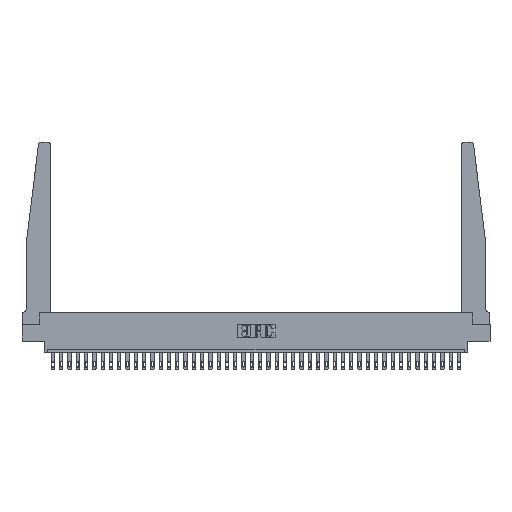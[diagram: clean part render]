
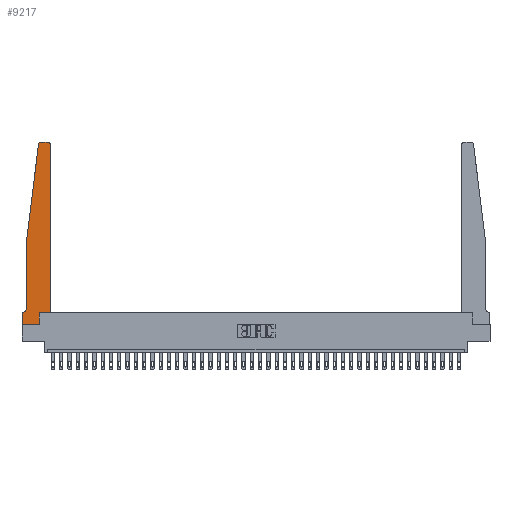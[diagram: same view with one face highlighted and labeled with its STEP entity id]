
A CAD part, top view. The second image highlights one B-rep face of the part: STEP entity #9217.
In plain terms, the highlighted planar face has unit normal (0, 0, 1).
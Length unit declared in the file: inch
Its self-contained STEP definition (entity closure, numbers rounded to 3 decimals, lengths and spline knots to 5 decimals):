
#181 = CARTESIAN_POINT ( 'NONE',  ( 0., 0.1875, 0.37 ) ) ;
#555 = LINE ( 'NONE', #16792, #15734 ) ;
#572 = VECTOR ( 'NONE', #16360, 39.37008 ) ;
#997 = CARTESIAN_POINT ( 'NONE',  ( 0.065, 1.25, 0.37 ) ) ;
#1011 = CARTESIAN_POINT ( 'NONE',  ( 0.065, 1.25, 0.37 ) ) ;
#1028 = EDGE_CURVE ( 'NONE', #31567, #10214, #10634, .T. ) ;
#1220 = CIRCLE ( 'NONE', #5780, 0.05 ) ;
#2375 = DIRECTION ( 'NONE',  ( 0., 0., 1. ) ) ;
#2556 = FACE_OUTER_BOUND ( 'NONE', #14897, .T. ) ;
#3318 = AXIS2_PLACEMENT_3D ( 'NONE', #9320, #3433, #23053 ) ;
#3376 = VERTEX_POINT ( 'NONE', #28971 ) ;
#3433 = DIRECTION ( 'NONE',  ( 0., 0., 1. ) ) ;
#4507 = LINE ( 'NONE', #18245, #8999 ) ;
#4530 = VECTOR ( 'NONE', #7963, 39.37008 ) ;
#4938 = EDGE_CURVE ( 'NONE', #9358, #31567, #4507, .T. ) ;
#5221 = CARTESIAN_POINT ( 'NONE',  ( 0.425, 2.72, 0.37 ) ) ;
#5393 = CARTESIAN_POINT ( 'NONE',  ( 0., 0.1875, 0.37 ) ) ;
#5651 = LINE ( 'NONE', #24561, #572 ) ;
#5780 = AXIS2_PLACEMENT_3D ( 'NONE', #29768, #18729, #18553 ) ;
#5893 = VERTEX_POINT ( 'NONE', #20055 ) ;
#6182 = ORIENTED_EDGE ( 'NONE', *, *, #1028, .T. ) ;
#6592 = EDGE_CURVE ( 'NONE', #24943, #9358, #1220, .T. ) ;
#7031 = VECTOR ( 'NONE', #18552, 39.37008 ) ;
#7167 = EDGE_CURVE ( 'NONE', #33819, #31018, #16520, .T. ) ;
#7266 = VERTEX_POINT ( 'NONE', #33075 ) ;
#7407 = VERTEX_POINT ( 'NONE', #25980 ) ;
#7668 = CARTESIAN_POINT ( 'NONE',  ( 0., 0., 0.37 ) ) ;
#7848 = LINE ( 'NONE', #7668, #7031 ) ;
#7963 = DIRECTION ( 'NONE',  ( -1., 0., 0. ) ) ;
#8357 = ORIENTED_EDGE ( 'NONE', *, *, #7167, .T. ) ;
#8999 = VECTOR ( 'NONE', #17708, 39.37008 ) ;
#9217 = ADVANCED_FACE ( 'NONE', ( #2556 ), #34974, .T. ) ;
#9297 = CARTESIAN_POINT ( 'NONE',  ( 0.065, 0.2375, 0.37 ) ) ;
#9320 = CARTESIAN_POINT ( 'NONE',  ( 0.27653, 2.72, 0.37 ) ) ;
#9358 = VERTEX_POINT ( 'NONE', #19488 ) ;
#9427 = DIRECTION ( 'NONE',  ( 0., -1., 0. ) ) ;
#9980 = ORIENTED_EDGE ( 'NONE', *, *, #11838, .T. ) ;
#10214 = VERTEX_POINT ( 'NONE', #28322 ) ;
#10397 = EDGE_CURVE ( 'NONE', #7266, #29901, #32520, .T. ) ;
#10634 = LINE ( 'NONE', #22047, #28386 ) ;
#11352 = DIRECTION ( 'NONE',  ( -0.122, -0.992, 0. ) ) ;
#11838 = EDGE_CURVE ( 'NONE', #5893, #7266, #5651, .T. ) ;
#12269 = LINE ( 'NONE', #28496, #30756 ) ;
#13611 = VECTOR ( 'NONE', #19169, 39.37008 ) ;
#14116 = AXIS2_PLACEMENT_3D ( 'NONE', #5393, #2375, #21468 ) ;
#14897 = EDGE_LOOP ( 'NONE', ( #18234, #28233, #8357, #33748, #35185, #18676, #6182, #30345, #31590, #9980, #26647, #16598 ) ) ;
#15734 = VECTOR ( 'NONE', #21629, 39.37008 ) ;
#16316 = CARTESIAN_POINT ( 'NONE',  ( 0.425, 0.18, 0.37 ) ) ;
#16360 = DIRECTION ( 'NONE',  ( 1., 0., 0. ) ) ;
#16520 = LINE ( 'NONE', #997, #17041 ) ;
#16598 = ORIENTED_EDGE ( 'NONE', *, *, #24276, .T. ) ;
#16792 = CARTESIAN_POINT ( 'NONE',  ( 0.2605, 0.18, 0.37 ) ) ;
#17041 = VECTOR ( 'NONE', #11352, 39.37008 ) ;
#17708 = DIRECTION ( 'NONE',  ( -1., 0., 0. ) ) ;
#18234 = ORIENTED_EDGE ( 'NONE', *, *, #32418, .T. ) ;
#18245 = CARTESIAN_POINT ( 'NONE',  ( 0.065, 0.1875, 0.37 ) ) ;
#18552 = DIRECTION ( 'NONE',  ( 1., 0., 0. ) ) ;
#18553 = DIRECTION ( 'NONE',  ( -1., 0., 0. ) ) ;
#18676 = ORIENTED_EDGE ( 'NONE', *, *, #4938, .T. ) ;
#18729 = DIRECTION ( 'NONE',  ( 0., 0., -1. ) ) ;
#19022 = AXIS2_PLACEMENT_3D ( 'NONE', #23329, #34876, #26531 ) ;
#19169 = DIRECTION ( 'NONE',  ( 0., 1., 0. ) ) ;
#19190 = DIRECTION ( 'NONE',  ( 0., -1., 0. ) ) ;
#19488 = CARTESIAN_POINT ( 'NONE',  ( 0.015, 0.1875, 0.37 ) ) ;
#20055 = CARTESIAN_POINT ( 'NONE',  ( 0.2605, 0.18, 0.37 ) ) ;
#20094 = CARTESIAN_POINT ( 'NONE',  ( 0.24675, 2.72367, 0.37 ) ) ;
#21468 = DIRECTION ( 'NONE',  ( 1., 0., 0. ) ) ;
#21629 = DIRECTION ( 'NONE',  ( 0., 1., 0. ) ) ;
#22047 = CARTESIAN_POINT ( 'NONE',  ( 0., 0., 0.37 ) ) ;
#22189 = CARTESIAN_POINT ( 'NONE',  ( 0.2605, 0., 0.37 ) ) ;
#23053 = DIRECTION ( 'NONE',  ( 1., 0., 0. ) ) ;
#23329 = CARTESIAN_POINT ( 'NONE',  ( 0.395, 2.72, 0.37 ) ) ;
#23921 = EDGE_CURVE ( 'NONE', #10214, #26660, #7848, .T. ) ;
#24276 = EDGE_CURVE ( 'NONE', #29901, #7407, #34361, .T. ) ;
#24561 = CARTESIAN_POINT ( 'NONE',  ( 0.425, 0.18, 0.37 ) ) ;
#24943 = VERTEX_POINT ( 'NONE', #9297 ) ;
#25980 = CARTESIAN_POINT ( 'NONE',  ( 0.395, 2.75, 0.37 ) ) ;
#26531 = DIRECTION ( 'NONE',  ( 1., 0., 0. ) ) ;
#26647 = ORIENTED_EDGE ( 'NONE', *, *, #10397, .T. ) ;
#26660 = VERTEX_POINT ( 'NONE', #22189 ) ;
#26694 = CIRCLE ( 'NONE', #3318, 0.03 ) ;
#27106 = EDGE_CURVE ( 'NONE', #26660, #5893, #555, .T. ) ;
#28233 = ORIENTED_EDGE ( 'NONE', *, *, #31314, .T. ) ;
#28322 = CARTESIAN_POINT ( 'NONE',  ( 0., 0., 0.37 ) ) ;
#28386 = VECTOR ( 'NONE', #19190, 39.37008 ) ;
#28496 = CARTESIAN_POINT ( 'NONE',  ( 0.065, 1.25, 0.37 ) ) ;
#28971 = CARTESIAN_POINT ( 'NONE',  ( 0.27653, 2.75, 0.37 ) ) ;
#29360 = LINE ( 'NONE', #32369, #4530 ) ;
#29768 = CARTESIAN_POINT ( 'NONE',  ( 0.015, 0.2375, 0.37 ) ) ;
#29901 = VERTEX_POINT ( 'NONE', #5221 ) ;
#30345 = ORIENTED_EDGE ( 'NONE', *, *, #23921, .T. ) ;
#30756 = VECTOR ( 'NONE', #9427, 39.37008 ) ;
#31018 = VERTEX_POINT ( 'NONE', #1011 ) ;
#31314 = EDGE_CURVE ( 'NONE', #3376, #33819, #26694, .T. ) ;
#31567 = VERTEX_POINT ( 'NONE', #181 ) ;
#31590 = ORIENTED_EDGE ( 'NONE', *, *, #27106, .T. ) ;
#32369 = CARTESIAN_POINT ( 'NONE',  ( 0.25, 2.75, 0.37 ) ) ;
#32418 = EDGE_CURVE ( 'NONE', #7407, #3376, #29360, .T. ) ;
#32520 = LINE ( 'NONE', #16316, #13611 ) ;
#33075 = CARTESIAN_POINT ( 'NONE',  ( 0.425, 0.18, 0.37 ) ) ;
#33525 = EDGE_CURVE ( 'NONE', #31018, #24943, #12269, .T. ) ;
#33748 = ORIENTED_EDGE ( 'NONE', *, *, #33525, .T. ) ;
#33819 = VERTEX_POINT ( 'NONE', #20094 ) ;
#34361 = CIRCLE ( 'NONE', #19022, 0.03 ) ;
#34876 = DIRECTION ( 'NONE',  ( 0., 0., 1. ) ) ;
#34974 = PLANE ( 'NONE',  #14116 ) ;
#35185 = ORIENTED_EDGE ( 'NONE', *, *, #6592, .T. ) ;
